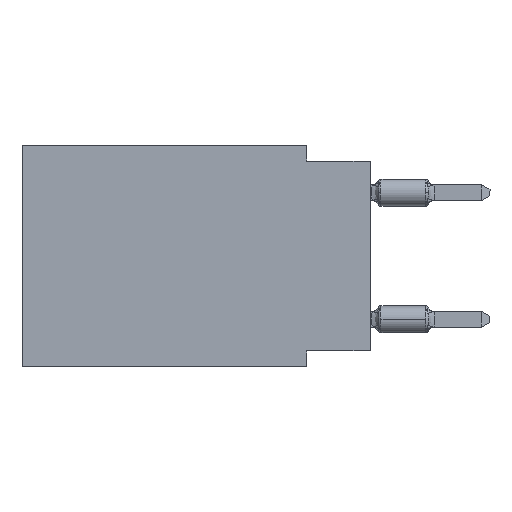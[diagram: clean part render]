
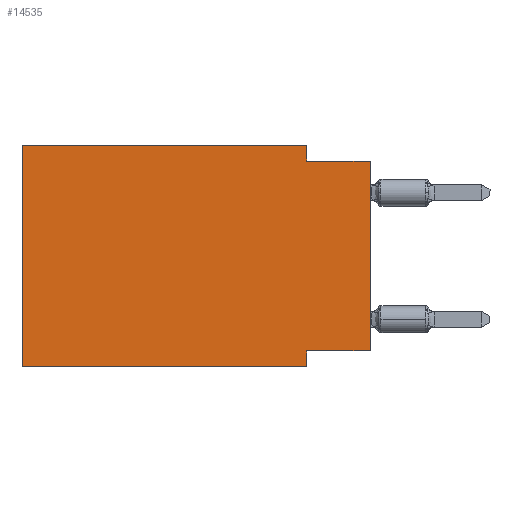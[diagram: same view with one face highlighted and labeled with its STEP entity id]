
A CAD part, left-side view. The second image highlights one B-rep face of the part: STEP entity #14535.
In plain terms, the highlighted planar face has unit normal (-1, 0, 0).
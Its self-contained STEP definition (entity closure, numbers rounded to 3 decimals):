
#287 = ORIENTED_EDGE ( 'NONE', *, *, #10481, .F. ) ;
#589 = CARTESIAN_POINT ( 'NONE',  ( 0., 13.97, 0. ) ) ;
#631 = LINE ( 'NONE', #10205, #1228 ) ;
#842 = ORIENTED_EDGE ( 'NONE', *, *, #10022, .T. ) ;
#893 = ORIENTED_EDGE ( 'NONE', *, *, #6962, .F. ) ;
#1228 = VECTOR ( 'NONE', #13575, 1000. ) ;
#1424 = PLANE ( 'NONE',  #5075 ) ;
#1646 = DIRECTION ( 'NONE',  ( 0., 0., -1. ) ) ;
#2380 = EDGE_CURVE ( 'NONE', #9362, #11854, #7683, .T. ) ;
#2515 = CARTESIAN_POINT ( 'NONE',  ( 0., 13.97, 0. ) ) ;
#2712 = CARTESIAN_POINT ( 'NONE',  ( 0., 13.97, -8.89 ) ) ;
#2853 = EDGE_CURVE ( 'NONE', #12836, #9930, #11329, .T. ) ;
#3070 = VECTOR ( 'NONE', #14124, 1000. ) ;
#3562 = VECTOR ( 'NONE', #9657, 1000. ) ;
#3662 = DIRECTION ( 'NONE',  ( 0., -1., 0. ) ) ;
#3722 = CARTESIAN_POINT ( 'NONE',  ( 0., 13.97, -8.89 ) ) ;
#4096 = ORIENTED_EDGE ( 'NONE', *, *, #2380, .F. ) ;
#4285 = EDGE_CURVE ( 'NONE', #12836, #13122, #6099, .T. ) ;
#5075 = AXIS2_PLACEMENT_3D ( 'NONE', #10973, #12231, #13172 ) ;
#5406 = DIRECTION ( 'NONE',  ( 0., 0., 1. ) ) ;
#5569 = CARTESIAN_POINT ( 'NONE',  ( 0., 2.54, -0.635 ) ) ;
#5689 = CARTESIAN_POINT ( 'NONE',  ( 0., 0., -8.255 ) ) ;
#5980 = CARTESIAN_POINT ( 'NONE',  ( 0., 0., 0. ) ) ;
#6099 = LINE ( 'NONE', #2712, #14725 ) ;
#6696 = EDGE_CURVE ( 'NONE', #7223, #13122, #631, .T. ) ;
#6962 = EDGE_CURVE ( 'NONE', #9930, #9362, #8626, .T. ) ;
#7223 = VERTEX_POINT ( 'NONE', #9248 ) ;
#7303 = DIRECTION ( 'NONE',  ( 0., -1., 0. ) ) ;
#7658 = LINE ( 'NONE', #7889, #15319 ) ;
#7683 = LINE ( 'NONE', #12372, #8628 ) ;
#7725 = CARTESIAN_POINT ( 'NONE',  ( 0., 2.54, 0. ) ) ;
#7889 = CARTESIAN_POINT ( 'NONE',  ( 0., 0., -0.635 ) ) ;
#8333 = EDGE_LOOP ( 'NONE', ( #842, #287, #4096, #893, #13991, #11073, #8582, #9139 ) ) ;
#8549 = VERTEX_POINT ( 'NONE', #10112 ) ;
#8582 = ORIENTED_EDGE ( 'NONE', *, *, #6696, .F. ) ;
#8626 = LINE ( 'NONE', #2515, #14022 ) ;
#8628 = VECTOR ( 'NONE', #1646, 1000. ) ;
#9139 = ORIENTED_EDGE ( 'NONE', *, *, #14339, .F. ) ;
#9248 = CARTESIAN_POINT ( 'NONE',  ( 0., 2.54, -8.255 ) ) ;
#9362 = VERTEX_POINT ( 'NONE', #7725 ) ;
#9657 = DIRECTION ( 'NONE',  ( 0., 0., 1. ) ) ;
#9930 = VERTEX_POINT ( 'NONE', #10373 ) ;
#10022 = EDGE_CURVE ( 'NONE', #8549, #12081, #13242, .T. ) ;
#10112 = CARTESIAN_POINT ( 'NONE',  ( 0., 0., -8.255 ) ) ;
#10143 = CARTESIAN_POINT ( 'NONE',  ( 0., 0., -0.635 ) ) ;
#10205 = CARTESIAN_POINT ( 'NONE',  ( 0., 2.54, -8.89 ) ) ;
#10373 = CARTESIAN_POINT ( 'NONE',  ( 0., 13.97, 0. ) ) ;
#10481 = EDGE_CURVE ( 'NONE', #11854, #12081, #7658, .T. ) ;
#10973 = CARTESIAN_POINT ( 'NONE',  ( 0., 13.97, 0. ) ) ;
#11073 = ORIENTED_EDGE ( 'NONE', *, *, #4285, .T. ) ;
#11329 = LINE ( 'NONE', #589, #13900 ) ;
#11768 = LINE ( 'NONE', #5689, #3070 ) ;
#11854 = VERTEX_POINT ( 'NONE', #5569 ) ;
#12081 = VERTEX_POINT ( 'NONE', #10143 ) ;
#12231 = DIRECTION ( 'NONE',  ( 1., 0., 0. ) ) ;
#12372 = CARTESIAN_POINT ( 'NONE',  ( 0., 2.54, 0. ) ) ;
#12420 = DIRECTION ( 'NONE',  ( 0., -1., 0. ) ) ;
#12836 = VERTEX_POINT ( 'NONE', #3722 ) ;
#13015 = CARTESIAN_POINT ( 'NONE',  ( 0., 2.54, -8.89 ) ) ;
#13122 = VERTEX_POINT ( 'NONE', #13015 ) ;
#13172 = DIRECTION ( 'NONE',  ( 0., 0., -1. ) ) ;
#13242 = LINE ( 'NONE', #5980, #3562 ) ;
#13575 = DIRECTION ( 'NONE',  ( 0., 0., -1. ) ) ;
#13900 = VECTOR ( 'NONE', #5406, 1000. ) ;
#13991 = ORIENTED_EDGE ( 'NONE', *, *, #2853, .F. ) ;
#14022 = VECTOR ( 'NONE', #7303, 1000. ) ;
#14124 = DIRECTION ( 'NONE',  ( 0., 1., 0. ) ) ;
#14339 = EDGE_CURVE ( 'NONE', #8549, #7223, #11768, .T. ) ;
#14535 = ADVANCED_FACE ( 'NONE', ( #14589 ), #1424, .F. ) ;
#14589 = FACE_OUTER_BOUND ( 'NONE', #8333, .T. ) ;
#14725 = VECTOR ( 'NONE', #3662, 1000. ) ;
#15319 = VECTOR ( 'NONE', #12420, 1000. ) ;
